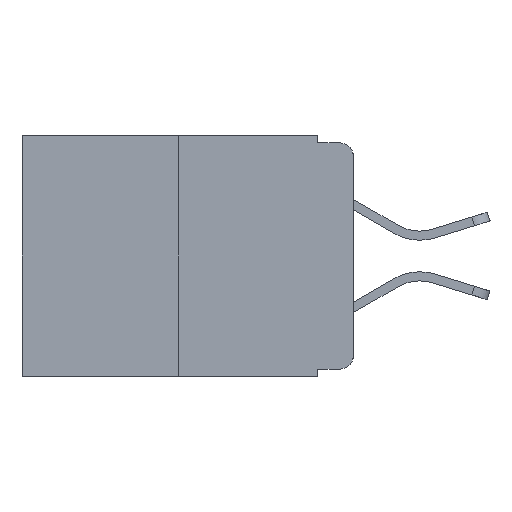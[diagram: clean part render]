
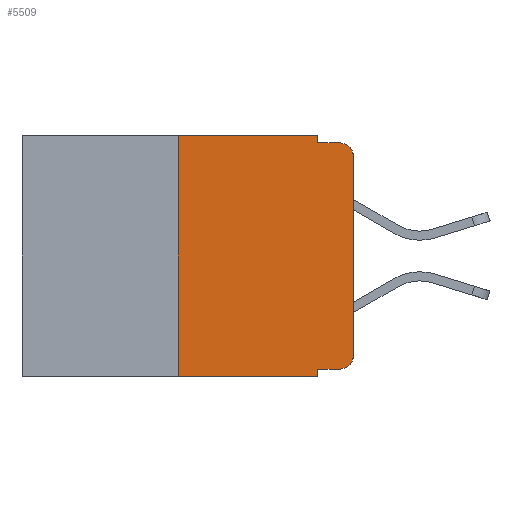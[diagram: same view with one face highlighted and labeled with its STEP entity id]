
A CAD part, left-side view. The second image highlights one B-rep face of the part: STEP entity #5509.
In plain terms, the highlighted planar face has unit normal (-1, 0, 0).
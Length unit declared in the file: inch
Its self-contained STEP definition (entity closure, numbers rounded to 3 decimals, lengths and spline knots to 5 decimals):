
#57 = VECTOR ( 'NONE', #20297, 39.37008 ) ;
#431 = VERTEX_POINT ( 'NONE', #12466 ) ;
#525 = CARTESIAN_POINT ( 'NONE',  ( 0., 0.051, -0.01 ) ) ;
#615 = CARTESIAN_POINT ( 'NONE',  ( 0., 0.473, 0. ) ) ;
#968 = AXIS2_PLACEMENT_3D ( 'NONE', #615, #17542, #17454 ) ;
#1203 = DIRECTION ( 'NONE',  ( 0., -1., 0. ) ) ;
#2969 = CARTESIAN_POINT ( 'NONE',  ( 0., 0.02, -0.01 ) ) ;
#3000 = DIRECTION ( 'NONE',  ( -1., 0., 0. ) ) ;
#3077 = DIRECTION ( 'NONE',  ( 0., 0., 1. ) ) ;
#3108 = ORIENTED_EDGE ( 'NONE', *, *, #15629, .F. ) ;
#3184 = CARTESIAN_POINT ( 'NONE',  ( 0., 0.25, -0.343 ) ) ;
#3548 = CARTESIAN_POINT ( 'NONE',  ( 0., 0.051, -0.333 ) ) ;
#4126 = AXIS2_PLACEMENT_3D ( 'NONE', #20477, #21965, #12669 ) ;
#4178 = EDGE_CURVE ( 'NONE', #12503, #431, #9879, .T. ) ;
#4435 = EDGE_CURVE ( 'NONE', #431, #11971, #5511, .T. ) ;
#4520 = VECTOR ( 'NONE', #23816, 39.37008 ) ;
#4779 = DIRECTION ( 'NONE',  ( 0., -1., 0. ) ) ;
#5396 = LINE ( 'NONE', #19847, #19994 ) ;
#5462 = FACE_OUTER_BOUND ( 'NONE', #9049, .T. ) ;
#5509 = ADVANCED_FACE ( 'NONE', ( #5462 ), #11816, .F. ) ;
#5511 = LINE ( 'NONE', #13649, #15732 ) ;
#5824 = LINE ( 'NONE', #7860, #13142 ) ;
#6328 = VERTEX_POINT ( 'NONE', #7014 ) ;
#6496 = EDGE_CURVE ( 'NONE', #23991, #16922, #5396, .T. ) ;
#6829 = ORIENTED_EDGE ( 'NONE', *, *, #4435, .F. ) ;
#7014 = CARTESIAN_POINT ( 'NONE',  ( 0., 0.02, -0.333 ) ) ;
#7709 = ORIENTED_EDGE ( 'NONE', *, *, #18384, .T. ) ;
#7860 = CARTESIAN_POINT ( 'NONE',  ( 0., 0.473, -0.343 ) ) ;
#7901 = EDGE_CURVE ( 'NONE', #9921, #24015, #10023, .T. ) ;
#8699 = LINE ( 'NONE', #10561, #19529 ) ;
#8740 = CARTESIAN_POINT ( 'NONE',  ( 0., 0., -0.313 ) ) ;
#9049 = EDGE_LOOP ( 'NONE', ( #22724, #17259, #15654, #3108, #6829, #13644, #17284, #10715, #12946, #7709 ) ) ;
#9879 = LINE ( 'NONE', #18461, #57 ) ;
#9921 = VERTEX_POINT ( 'NONE', #3548 ) ;
#10023 = LINE ( 'NONE', #12578, #4520 ) ;
#10174 = CIRCLE ( 'NONE', #4126, 0.02 ) ;
#10561 = CARTESIAN_POINT ( 'NONE',  ( 0., 0.051, -0.333 ) ) ;
#10715 = ORIENTED_EDGE ( 'NONE', *, *, #7901, .F. ) ;
#11237 = VECTOR ( 'NONE', #22377, 39.37008 ) ;
#11630 = DIRECTION ( 'NONE',  ( 0., -1., 0. ) ) ;
#11816 = PLANE ( 'NONE',  #968 ) ;
#11971 = VERTEX_POINT ( 'NONE', #19493 ) ;
#12142 = AXIS2_PLACEMENT_3D ( 'NONE', #21625, #3000, #13975 ) ;
#12466 = CARTESIAN_POINT ( 'NONE',  ( 0., 0.25, 0. ) ) ;
#12503 = VERTEX_POINT ( 'NONE', #3184 ) ;
#12573 = VERTEX_POINT ( 'NONE', #8740 ) ;
#12578 = CARTESIAN_POINT ( 'NONE',  ( 0., 0.051, 0. ) ) ;
#12669 = DIRECTION ( 'NONE',  ( 0., 0., -1. ) ) ;
#12946 = ORIENTED_EDGE ( 'NONE', *, *, #17564, .T. ) ;
#13142 = VECTOR ( 'NONE', #11630, 39.37008 ) ;
#13160 = EDGE_CURVE ( 'NONE', #12573, #17906, #22986, .T. ) ;
#13192 = EDGE_CURVE ( 'NONE', #17906, #16922, #16009, .T. ) ;
#13644 = ORIENTED_EDGE ( 'NONE', *, *, #4178, .F. ) ;
#13649 = CARTESIAN_POINT ( 'NONE',  ( 0., 0.473, 0. ) ) ;
#13776 = CARTESIAN_POINT ( 'NONE',  ( 0., 0.051, -0.343 ) ) ;
#13975 = DIRECTION ( 'NONE',  ( 0., 0., -1. ) ) ;
#14718 = CARTESIAN_POINT ( 'NONE',  ( 0., 0.051, 0. ) ) ;
#15214 = CARTESIAN_POINT ( 'NONE',  ( 0., 0., -0.03 ) ) ;
#15629 = EDGE_CURVE ( 'NONE', #11971, #23991, #21171, .T. ) ;
#15654 = ORIENTED_EDGE ( 'NONE', *, *, #6496, .F. ) ;
#15732 = VECTOR ( 'NONE', #1203, 39.37008 ) ;
#16009 = CIRCLE ( 'NONE', #12142, 0.02 ) ;
#16922 = VERTEX_POINT ( 'NONE', #2969 ) ;
#17243 = EDGE_CURVE ( 'NONE', #12503, #24015, #5824, .T. ) ;
#17259 = ORIENTED_EDGE ( 'NONE', *, *, #13192, .T. ) ;
#17284 = ORIENTED_EDGE ( 'NONE', *, *, #17243, .T. ) ;
#17454 = DIRECTION ( 'NONE',  ( 0., 0., -1. ) ) ;
#17542 = DIRECTION ( 'NONE',  ( 1., 0., 0. ) ) ;
#17564 = EDGE_CURVE ( 'NONE', #9921, #6328, #8699, .T. ) ;
#17779 = DIRECTION ( 'NONE',  ( 0., -1., 0. ) ) ;
#17906 = VERTEX_POINT ( 'NONE', #15214 ) ;
#18384 = EDGE_CURVE ( 'NONE', #6328, #12573, #10174, .T. ) ;
#18461 = CARTESIAN_POINT ( 'NONE',  ( 0., 0.25, 0. ) ) ;
#19493 = CARTESIAN_POINT ( 'NONE',  ( 0., 0.051, 0. ) ) ;
#19529 = VECTOR ( 'NONE', #17779, 39.37008 ) ;
#19839 = CARTESIAN_POINT ( 'NONE',  ( 0., 0., 0. ) ) ;
#19847 = CARTESIAN_POINT ( 'NONE',  ( 0., 0.051, -0.01 ) ) ;
#19994 = VECTOR ( 'NONE', #4779, 39.37008 ) ;
#20297 = DIRECTION ( 'NONE',  ( 0., 0., 1. ) ) ;
#20477 = CARTESIAN_POINT ( 'NONE',  ( 0., 0.02, -0.313 ) ) ;
#21171 = LINE ( 'NONE', #14718, #11237 ) ;
#21625 = CARTESIAN_POINT ( 'NONE',  ( 0., 0.02, -0.03 ) ) ;
#21965 = DIRECTION ( 'NONE',  ( -1., 0., 0. ) ) ;
#22377 = DIRECTION ( 'NONE',  ( 0., 0., -1. ) ) ;
#22724 = ORIENTED_EDGE ( 'NONE', *, *, #13160, .T. ) ;
#22986 = LINE ( 'NONE', #19839, #23883 ) ;
#23816 = DIRECTION ( 'NONE',  ( 0., 0., -1. ) ) ;
#23883 = VECTOR ( 'NONE', #3077, 39.37008 ) ;
#23991 = VERTEX_POINT ( 'NONE', #525 ) ;
#24015 = VERTEX_POINT ( 'NONE', #13776 ) ;
